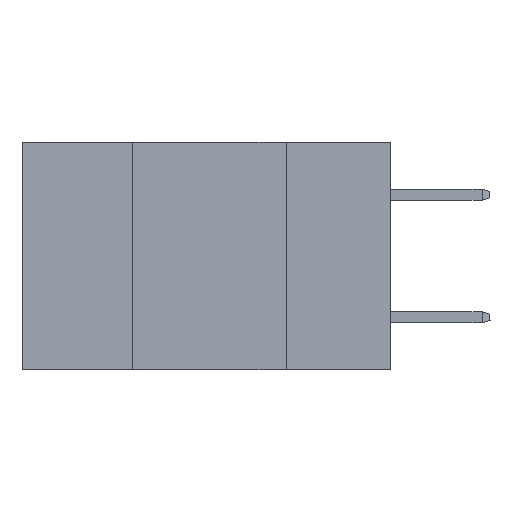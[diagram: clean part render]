
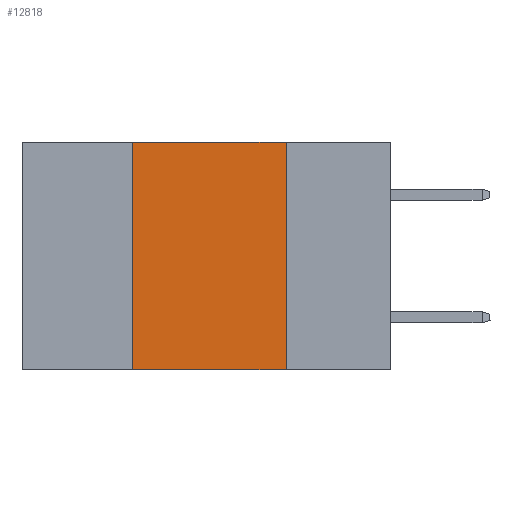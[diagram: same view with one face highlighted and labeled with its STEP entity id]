
A CAD part, left-side view. The second image highlights one B-rep face of the part: STEP entity #12818.
In plain terms, the highlighted planar face has unit normal (-1, 0, 0).
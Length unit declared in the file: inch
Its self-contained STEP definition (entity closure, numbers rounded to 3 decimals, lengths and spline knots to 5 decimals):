
#709 = LINE ( 'NONE', #20911, #2701 ) ;
#2701 = VECTOR ( 'NONE', #26236, 39.37008 ) ;
#3823 = DIRECTION ( 'NONE',  ( 0., 0., -1. ) ) ;
#6070 = VERTEX_POINT ( 'NONE', #18492 ) ;
#6781 = VERTEX_POINT ( 'NONE', #14846 ) ;
#7796 = DIRECTION ( 'NONE',  ( 0., 0., -1. ) ) ;
#9092 = CARTESIAN_POINT ( 'NONE',  ( 0., 0.42, 0. ) ) ;
#9426 = DIRECTION ( 'NONE',  ( 0., 0., 1. ) ) ;
#10550 = LINE ( 'NONE', #30239, #14000 ) ;
#12818 = ADVANCED_FACE ( 'NONE', ( #22969 ), #20473, .F. ) ;
#13076 = VERTEX_POINT ( 'NONE', #21944 ) ;
#13295 = DIRECTION ( 'NONE',  ( 1., 0., 0. ) ) ;
#14000 = VECTOR ( 'NONE', #3823, 39.37008 ) ;
#14637 = ORIENTED_EDGE ( 'NONE', *, *, #23628, .F. ) ;
#14846 = CARTESIAN_POINT ( 'NONE',  ( 0., 0.17, 0. ) ) ;
#15237 = EDGE_CURVE ( 'NONE', #13076, #31401, #709, .T. ) ;
#15978 = ORIENTED_EDGE ( 'NONE', *, *, #15237, .T. ) ;
#16346 = VECTOR ( 'NONE', #9426, 39.37008 ) ;
#16999 = EDGE_CURVE ( 'NONE', #6781, #31401, #10550, .T. ) ;
#18492 = CARTESIAN_POINT ( 'NONE',  ( 0., 0.42, 0. ) ) ;
#20473 = PLANE ( 'NONE',  #21241 ) ;
#20911 = CARTESIAN_POINT ( 'NONE',  ( 0., 0.6, -0.37 ) ) ;
#21241 = AXIS2_PLACEMENT_3D ( 'NONE', #30826, #13295, #7796 ) ;
#21599 = ORIENTED_EDGE ( 'NONE', *, *, #27202, .F. ) ;
#21944 = CARTESIAN_POINT ( 'NONE',  ( 0., 0.42, -0.37 ) ) ;
#22969 = FACE_OUTER_BOUND ( 'NONE', #32286, .T. ) ;
#23228 = ORIENTED_EDGE ( 'NONE', *, *, #16999, .F. ) ;
#23628 = EDGE_CURVE ( 'NONE', #13076, #6070, #31950, .T. ) ;
#24699 = CARTESIAN_POINT ( 'NONE',  ( 0., 0.6, 0. ) ) ;
#25052 = CARTESIAN_POINT ( 'NONE',  ( 0., 0.17, -0.37 ) ) ;
#26236 = DIRECTION ( 'NONE',  ( 0., -1., 0. ) ) ;
#27202 = EDGE_CURVE ( 'NONE', #6070, #6781, #27524, .T. ) ;
#27524 = LINE ( 'NONE', #24699, #29298 ) ;
#29298 = VECTOR ( 'NONE', #32212, 39.37008 ) ;
#30239 = CARTESIAN_POINT ( 'NONE',  ( 0., 0.17, 0. ) ) ;
#30826 = CARTESIAN_POINT ( 'NONE',  ( 0., 0.6, 0. ) ) ;
#31401 = VERTEX_POINT ( 'NONE', #25052 ) ;
#31950 = LINE ( 'NONE', #9092, #16346 ) ;
#32212 = DIRECTION ( 'NONE',  ( 0., -1., 0. ) ) ;
#32286 = EDGE_LOOP ( 'NONE', ( #23228, #21599, #14637, #15978 ) ) ;
